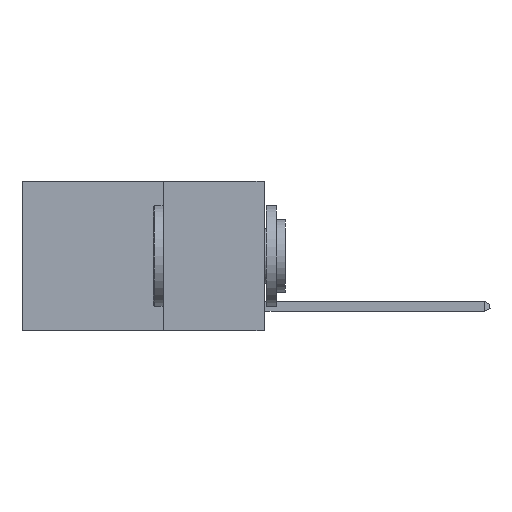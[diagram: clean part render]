
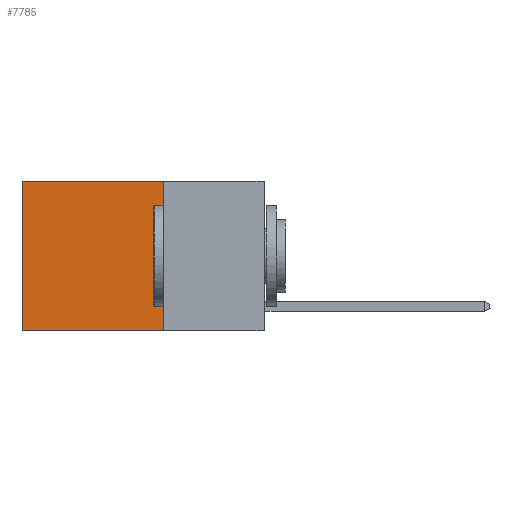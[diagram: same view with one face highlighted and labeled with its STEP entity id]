
A CAD part, left-side view. The second image highlights one B-rep face of the part: STEP entity #7785.
In plain terms, the highlighted planar face has unit normal (-1, 0, 0).
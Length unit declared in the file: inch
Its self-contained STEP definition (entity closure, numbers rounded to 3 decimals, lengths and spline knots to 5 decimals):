
#312 = EDGE_CURVE ( 'NONE', #9210, #1564, #4710, .T. ) ;
#459 = CARTESIAN_POINT ( 'NONE',  ( 0.2625, 0.25, -0.37 ) ) ;
#593 = EDGE_CURVE ( 'NONE', #9210, #4970, #2773, .T. ) ;
#911 = VECTOR ( 'NONE', #9498, 39.37008 ) ;
#1207 = CARTESIAN_POINT ( 'NONE',  ( 0.2625, 0.25, 0. ) ) ;
#1272 = CARTESIAN_POINT ( 'NONE',  ( 0.2625, 0.6, 0. ) ) ;
#1411 = CARTESIAN_POINT ( 'NONE',  ( 0.2625, 0.25, 0. ) ) ;
#1423 = ORIENTED_EDGE ( 'NONE', *, *, #312, .T. ) ;
#1495 = CARTESIAN_POINT ( 'NONE',  ( 0.2625, 0.6, 0. ) ) ;
#1537 = VERTEX_POINT ( 'NONE', #2243 ) ;
#1564 = VERTEX_POINT ( 'NONE', #1272 ) ;
#2170 = DIRECTION ( 'NONE',  ( 0., 1., 0. ) ) ;
#2243 = CARTESIAN_POINT ( 'NONE',  ( 0.2625, 0.6, -0.37 ) ) ;
#2475 = ORIENTED_EDGE ( 'NONE', *, *, #593, .F. ) ;
#2773 = LINE ( 'NONE', #1207, #10746 ) ;
#3246 = EDGE_CURVE ( 'NONE', #4970, #1537, #7584, .T. ) ;
#3421 = LINE ( 'NONE', #1495, #10730 ) ;
#4710 = LINE ( 'NONE', #10287, #11097 ) ;
#4970 = VERTEX_POINT ( 'NONE', #459 ) ;
#5578 = EDGE_CURVE ( 'NONE', #1564, #1537, #3421, .T. ) ;
#5634 = CARTESIAN_POINT ( 'NONE',  ( 0.2625, 0.25, -0.37 ) ) ;
#6028 = FACE_OUTER_BOUND ( 'NONE', #11139, .T. ) ;
#6395 = ORIENTED_EDGE ( 'NONE', *, *, #5578, .T. ) ;
#6702 = DIRECTION ( 'NONE',  ( 0., 0., -1. ) ) ;
#6739 = PLANE ( 'NONE',  #8145 ) ;
#7167 = CARTESIAN_POINT ( 'NONE',  ( 0.2625, 0.25, 0. ) ) ;
#7584 = LINE ( 'NONE', #5634, #911 ) ;
#7785 = ADVANCED_FACE ( 'NONE', ( #6028 ), #6739, .F. ) ;
#8145 = AXIS2_PLACEMENT_3D ( 'NONE', #1411, #10533, #9669 ) ;
#9210 = VERTEX_POINT ( 'NONE', #7167 ) ;
#9498 = DIRECTION ( 'NONE',  ( 0., 1., 0. ) ) ;
#9669 = DIRECTION ( 'NONE',  ( 0., 0., -1. ) ) ;
#10287 = CARTESIAN_POINT ( 'NONE',  ( 0.2625, 0.25, 0. ) ) ;
#10334 = ORIENTED_EDGE ( 'NONE', *, *, #3246, .F. ) ;
#10533 = DIRECTION ( 'NONE',  ( 1., 0., 0. ) ) ;
#10730 = VECTOR ( 'NONE', #11413, 39.37008 ) ;
#10746 = VECTOR ( 'NONE', #6702, 39.37008 ) ;
#11097 = VECTOR ( 'NONE', #2170, 39.37008 ) ;
#11139 = EDGE_LOOP ( 'NONE', ( #6395, #10334, #2475, #1423 ) ) ;
#11413 = DIRECTION ( 'NONE',  ( 0., 0., -1. ) ) ;
